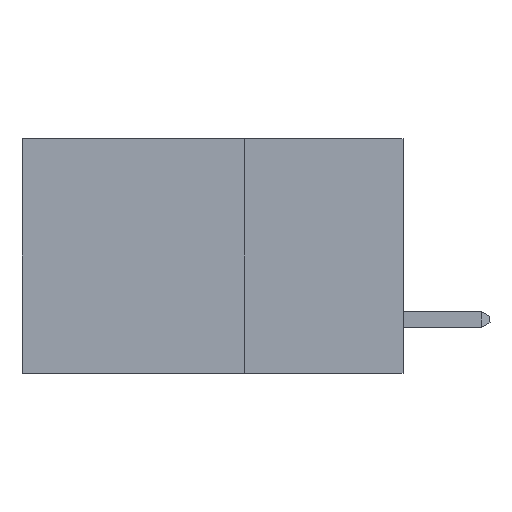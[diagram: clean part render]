
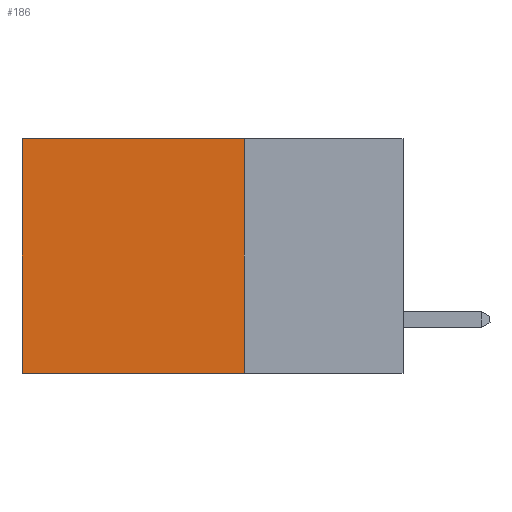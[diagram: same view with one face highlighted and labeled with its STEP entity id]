
A CAD part, left-side view. The second image highlights one B-rep face of the part: STEP entity #186.
In plain terms, the highlighted planar face has unit normal (-1, 0, 0).
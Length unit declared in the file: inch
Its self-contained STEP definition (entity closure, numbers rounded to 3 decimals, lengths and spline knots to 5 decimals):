
#164 = EDGE_CURVE ( 'NONE', #1039, #9583, #11124, .T. ) ;
#186 = ADVANCED_FACE ( 'NONE', ( #10233 ), #5902, .F. ) ;
#473 = CARTESIAN_POINT ( 'NONE',  ( 0.2875, 0.25, -0.37 ) ) ;
#518 = CARTESIAN_POINT ( 'NONE',  ( 0.2875, 0.25, 0. ) ) ;
#838 = CARTESIAN_POINT ( 'NONE',  ( 0.2875, 0.6, -0.37 ) ) ;
#1039 = VERTEX_POINT ( 'NONE', #7814 ) ;
#1521 = VERTEX_POINT ( 'NONE', #518 ) ;
#1982 = EDGE_CURVE ( 'NONE', #1521, #4587, #3081, .T. ) ;
#2319 = CARTESIAN_POINT ( 'NONE',  ( 0.2875, 0.25, 0. ) ) ;
#3081 = LINE ( 'NONE', #6368, #6149 ) ;
#3333 = LINE ( 'NONE', #2319, #11019 ) ;
#4587 = VERTEX_POINT ( 'NONE', #473 ) ;
#5069 = DIRECTION ( 'NONE',  ( 0., 0., -1. ) ) ;
#5223 = VECTOR ( 'NONE', #5069, 39.37008 ) ;
#5308 = ORIENTED_EDGE ( 'NONE', *, *, #7744, .F. ) ;
#5902 = PLANE ( 'NONE',  #12199 ) ;
#6149 = VECTOR ( 'NONE', #6907, 39.37008 ) ;
#6368 = CARTESIAN_POINT ( 'NONE',  ( 0.2875, 0.25, 0. ) ) ;
#6907 = DIRECTION ( 'NONE',  ( 0., 0., -1. ) ) ;
#7246 = EDGE_LOOP ( 'NONE', ( #10427, #5308, #9862, #7255 ) ) ;
#7255 = ORIENTED_EDGE ( 'NONE', *, *, #8062, .T. ) ;
#7462 = CARTESIAN_POINT ( 'NONE',  ( 0.2875, 0.6, 0. ) ) ;
#7744 = EDGE_CURVE ( 'NONE', #4587, #9583, #10425, .T. ) ;
#7814 = CARTESIAN_POINT ( 'NONE',  ( 0.2875, 0.6, 0. ) ) ;
#7856 = VECTOR ( 'NONE', #11835, 39.37008 ) ;
#8062 = EDGE_CURVE ( 'NONE', #1521, #1039, #3333, .T. ) ;
#8924 = CARTESIAN_POINT ( 'NONE',  ( 0.2875, 0.25, -0.37 ) ) ;
#9583 = VERTEX_POINT ( 'NONE', #838 ) ;
#9862 = ORIENTED_EDGE ( 'NONE', *, *, #1982, .F. ) ;
#10233 = FACE_OUTER_BOUND ( 'NONE', #7246, .T. ) ;
#10399 = DIRECTION ( 'NONE',  ( 0., 1., 0. ) ) ;
#10425 = LINE ( 'NONE', #8924, #7856 ) ;
#10427 = ORIENTED_EDGE ( 'NONE', *, *, #164, .T. ) ;
#11019 = VECTOR ( 'NONE', #10399, 39.37008 ) ;
#11029 = CARTESIAN_POINT ( 'NONE',  ( 0.2875, 0.25, 0. ) ) ;
#11124 = LINE ( 'NONE', #7462, #5223 ) ;
#11835 = DIRECTION ( 'NONE',  ( 0., 1., 0. ) ) ;
#12199 = AXIS2_PLACEMENT_3D ( 'NONE', #11029, #12960, #12909 ) ;
#12909 = DIRECTION ( 'NONE',  ( 0., 0., -1. ) ) ;
#12960 = DIRECTION ( 'NONE',  ( 1., 0., 0. ) ) ;
